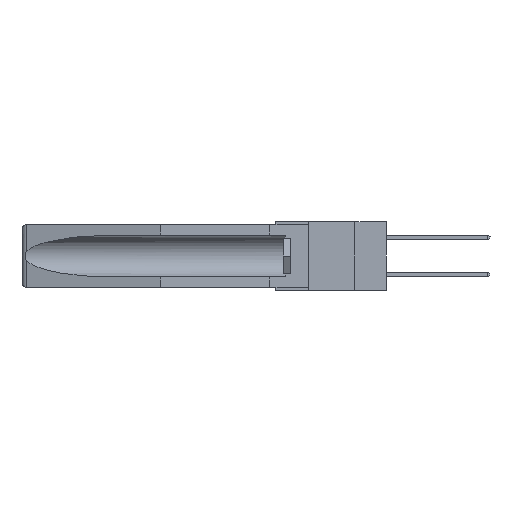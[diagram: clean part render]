
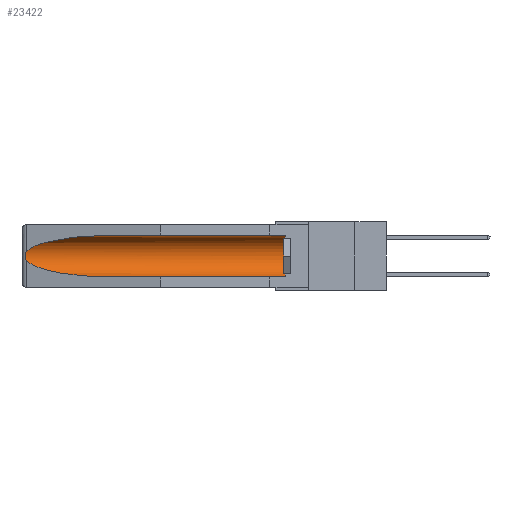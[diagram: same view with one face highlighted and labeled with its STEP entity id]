
A CAD part, left-side view. The second image highlights one B-rep face of the part: STEP entity #23422.
In plain terms, the highlighted cylindrical face has radius 2.857 mm (diameter 5.715 mm), a partial arc.
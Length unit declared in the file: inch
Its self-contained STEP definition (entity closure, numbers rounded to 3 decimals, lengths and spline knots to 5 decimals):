
#523 = CARTESIAN_POINT ( 'NONE',  ( 0.155, 0.126, -0.1715 ) ) ;
#698 = AXIS2_PLACEMENT_3D ( 'NONE', #8453, #717, #23789 ) ;
#717 = DIRECTION ( 'NONE',  ( 0., 1., 0. ) ) ;
#948 = CARTESIAN_POINT ( 'NONE',  ( 0.155, 1.07973, -0.284 ) ) ;
#1041 = CARTESIAN_POINT ( 'NONE',  ( 0.155, 1.07973, -0.059 ) ) ;
#1070 = CARTESIAN_POINT ( 'NONE',  ( 0.26537, 1.52718, -0.19328 ) ) ;
#1121 = CARTESIAN_POINT ( 'NONE',  ( 0.26537, 1.52718, -0.14972 ) ) ;
#1165 = EDGE_CURVE ( 'NONE', #15055, #21548, #23312, .T. ) ;
#1959 = VERTEX_POINT ( 'NONE', #14268 ) ;
#2710 = CYLINDRICAL_SURFACE ( 'NONE', #698, 0.1125 ) ;
#2791 = ORIENTED_EDGE ( 'NONE', *, *, #8812, .T. ) ;
#2996 = CARTESIAN_POINT ( 'NONE',  ( 0.21114, 1.30732, -0.284 ) ) ;
#3769 = ORIENTED_EDGE ( 'NONE', *, *, #6893, .F. ) ;
#4225 = CIRCLE ( 'NONE', #7591, 0.1125 ) ;
#4752 = CARTESIAN_POINT ( 'NONE',  ( 0.21114, 1.30732, -0.059 ) ) ;
#5656 = VECTOR ( 'NONE', #10652, 39.37008 ) ;
#5957 =( BOUNDED_CURVE ( )  B_SPLINE_CURVE ( 3, ( #1070, #10533, #2996, #20196 ),
 .UNSPECIFIED., .F., .F. ) 
 B_SPLINE_CURVE_WITH_KNOTS ( ( 4, 4 ),
 ( 0.1948, 1.5708 ),
 .UNSPECIFIED. ) 
 CURVE ( )  GEOMETRIC_REPRESENTATION_ITEM ( )  RATIONAL_B_SPLINE_CURVE ( ( 1., 0.848, 0.848, 1. ) ) 
 REPRESENTATION_ITEM ( '' )  );
#6291 = CARTESIAN_POINT ( 'NONE',  ( 0.155, 0.126, -0.059 ) ) ;
#6839 = CARTESIAN_POINT ( 'NONE',  ( 0.25451, 1.48313, -0.09465 ) ) ;
#6893 = EDGE_CURVE ( 'NONE', #20076, #13832, #18204, .T. ) ;
#7051 = CARTESIAN_POINT ( 'NONE',  ( 0.26654, 1.53092, -0.15636 ) ) ;
#7124 = CARTESIAN_POINT ( 'NONE',  ( 0.2675, 1.53308, -0.17534 ) ) ;
#7591 = AXIS2_PLACEMENT_3D ( 'NONE', #523, #19570, #12173 ) ;
#8091 = ORIENTED_EDGE ( 'NONE', *, *, #20545, .T. ) ;
#8453 = CARTESIAN_POINT ( 'NONE',  ( 0.155, -0.30754, -0.1715 ) ) ;
#8526 = CARTESIAN_POINT ( 'NONE',  ( 0.26537, 1.52718, -0.14972 ) ) ;
#8596 = CARTESIAN_POINT ( 'NONE',  ( 0.155, -0.30754, -0.059 ) ) ;
#8812 = EDGE_CURVE ( 'NONE', #21548, #1959, #24086, .T. ) ;
#9061 = CARTESIAN_POINT ( 'NONE',  ( 0.2673, 1.53269, -0.17917 ) ) ;
#10301 = CARTESIAN_POINT ( 'NONE',  ( 0.155, 0.126, -0.284 ) ) ;
#10533 = CARTESIAN_POINT ( 'NONE',  ( 0.25451, 1.48313, -0.24835 ) ) ;
#10629 = CARTESIAN_POINT ( 'NONE',  ( 0.26597, 1.5296, -0.19026 ) ) ;
#10652 = DIRECTION ( 'NONE',  ( 0., 1., 0. ) ) ;
#11506 = CARTESIAN_POINT ( 'NONE',  ( 0.155, 1.07973, -0.059 ) ) ;
#12173 = DIRECTION ( 'NONE',  ( 0., 0., 1. ) ) ;
#12189 = VECTOR ( 'NONE', #13909, 39.37008 ) ;
#12566 = CARTESIAN_POINT ( 'NONE',  ( 0.26537, 1.52718, -0.19328 ) ) ;
#12806 = CARTESIAN_POINT ( 'NONE',  ( 0.26597, 1.52961, -0.15275 ) ) ;
#13447 = ORIENTED_EDGE ( 'NONE', *, *, #16054, .T. ) ;
#13832 = VERTEX_POINT ( 'NONE', #948 ) ;
#13909 = DIRECTION ( 'NONE',  ( 0., 1., 0. ) ) ;
#14031 = LINE ( 'NONE', #8596, #5656 ) ;
#14268 = CARTESIAN_POINT ( 'NONE',  ( 0.26537, 1.52718, -0.19328 ) ) ;
#14422 = CARTESIAN_POINT ( 'NONE',  ( 0.26655, 1.53094, -0.18657 ) ) ;
#15055 = VERTEX_POINT ( 'NONE', #11506 ) ;
#16054 = EDGE_CURVE ( 'NONE', #1959, #13832, #5957, .T. ) ;
#17089 = EDGE_LOOP ( 'NONE', ( #20797, #2791, #13447, #3769, #8091, #22187 ) ) ;
#18204 = LINE ( 'NONE', #23473, #12189 ) ;
#18291 = CARTESIAN_POINT ( 'NONE',  ( 0.2675, 1.53308, -0.16763 ) ) ;
#18539 = CARTESIAN_POINT ( 'NONE',  ( 0.26537, 1.52718, -0.14972 ) ) ;
#19570 = DIRECTION ( 'NONE',  ( 0., -1., 0. ) ) ;
#20076 = VERTEX_POINT ( 'NONE', #10301 ) ;
#20196 = CARTESIAN_POINT ( 'NONE',  ( 0.155, 1.07973, -0.284 ) ) ;
#20466 = CARTESIAN_POINT ( 'NONE',  ( 0.2673, 1.5327, -0.16383 ) ) ;
#20545 = EDGE_CURVE ( 'NONE', #20076, #23285, #4225, .T. ) ;
#20797 = ORIENTED_EDGE ( 'NONE', *, *, #1165, .T. ) ;
#21548 = VERTEX_POINT ( 'NONE', #1121 ) ;
#22187 = ORIENTED_EDGE ( 'NONE', *, *, #22732, .T. ) ;
#22732 = EDGE_CURVE ( 'NONE', #23285, #15055, #14031, .T. ) ;
#23285 = VERTEX_POINT ( 'NONE', #6291 ) ;
#23312 =( BOUNDED_CURVE ( )  B_SPLINE_CURVE ( 3, ( #1041, #4752, #6839, #8526 ),
 .UNSPECIFIED., .F., .F. ) 
 B_SPLINE_CURVE_WITH_KNOTS ( ( 4, 4 ),
 ( 4.71239, 6.08839 ),
 .UNSPECIFIED. ) 
 CURVE ( )  GEOMETRIC_REPRESENTATION_ITEM ( )  RATIONAL_B_SPLINE_CURVE ( ( 1., 0.848, 0.848, 1. ) ) 
 REPRESENTATION_ITEM ( '' )  );
#23422 = ADVANCED_FACE ( 'NONE', ( #23715 ), #2710, .F. ) ;
#23473 = CARTESIAN_POINT ( 'NONE',  ( 0.155, -0.30754, -0.284 ) ) ;
#23715 = FACE_OUTER_BOUND ( 'NONE', #17089, .T. ) ;
#23789 = DIRECTION ( 'NONE',  ( 0., 0., 1. ) ) ;
#24086 = B_SPLINE_CURVE_WITH_KNOTS ( 'NONE', 3,
 ( #18539, #12806, #7051, #20466, #18291, #7124, #9061, #14422, #10629, #12566 ),
 .UNSPECIFIED., .F., .F.,
 ( 4, 2, 2, 2, 4 ),
 ( 0., 0.00029, 0.00058, 0.00087, 0.00117 ),
 .UNSPECIFIED. ) ;
